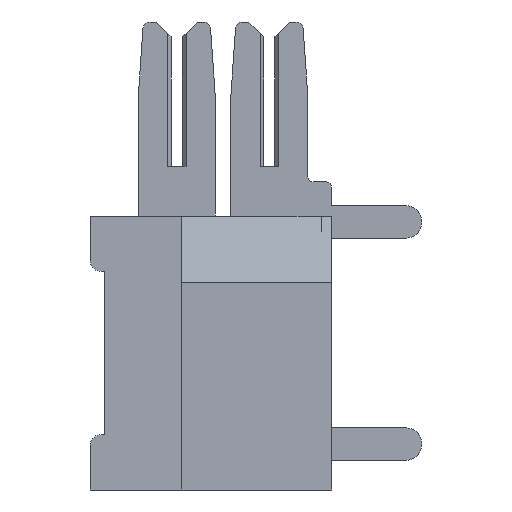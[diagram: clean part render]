
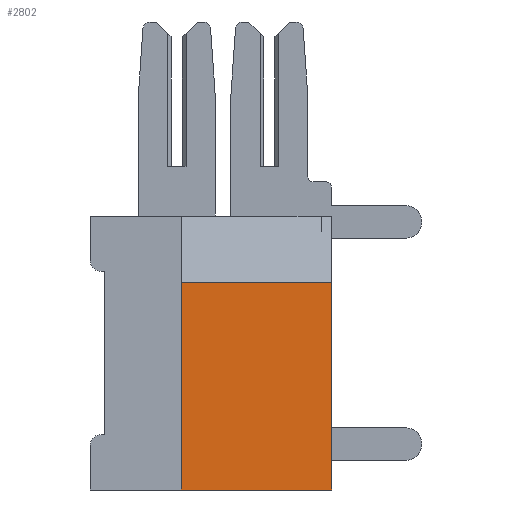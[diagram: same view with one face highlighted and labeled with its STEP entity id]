
A CAD part, left-side view. The second image highlights one B-rep face of the part: STEP entity #2802.
In plain terms, the highlighted planar face has unit normal (-1, 0, 0).
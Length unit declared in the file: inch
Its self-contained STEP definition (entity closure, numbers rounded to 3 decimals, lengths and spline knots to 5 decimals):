
#1 = FACE_OUTER_BOUND ( 'NONE', #800, .T. ) ;
#390 = CARTESIAN_POINT ( 'NONE',  ( 0., 0.326, 0. ) ) ;
#412 = VECTOR ( 'NONE', #3833, 39.37008 ) ;
#800 = EDGE_LOOP ( 'NONE', ( #5650, #11852, #9499, #2534 ) ) ;
#1183 = VERTEX_POINT ( 'NONE', #2715 ) ;
#1211 = EDGE_CURVE ( 'NONE', #10266, #1183, #1977, .T. ) ;
#1630 = DIRECTION ( 'NONE',  ( 0., -1., 0. ) ) ;
#1977 = LINE ( 'NONE', #2856, #8263 ) ;
#2450 = DIRECTION ( 'NONE',  ( 1., 0., 0. ) ) ;
#2514 = LINE ( 'NONE', #2945, #10423 ) ;
#2534 = ORIENTED_EDGE ( 'NONE', *, *, #1211, .T. ) ;
#2715 = CARTESIAN_POINT ( 'NONE',  ( 0., 0., -0.37 ) ) ;
#2802 = ADVANCED_FACE ( 'NONE', ( #1 ), #12447, .F. ) ;
#2856 = CARTESIAN_POINT ( 'NONE',  ( 0., 0.326, -0.37 ) ) ;
#2945 = CARTESIAN_POINT ( 'NONE',  ( 0., 0., -0.09 ) ) ;
#3150 = LINE ( 'NONE', #8929, #412 ) ;
#3765 = AXIS2_PLACEMENT_3D ( 'NONE', #390, #2450, #12671 ) ;
#3833 = DIRECTION ( 'NONE',  ( 0., 0., 1. ) ) ;
#4288 = VERTEX_POINT ( 'NONE', #12915 ) ;
#5051 = DIRECTION ( 'NONE',  ( 0., 1., 0. ) ) ;
#5117 = DIRECTION ( 'NONE',  ( 0., 0., 1. ) ) ;
#5650 = ORIENTED_EDGE ( 'NONE', *, *, #12595, .T. ) ;
#6531 = LINE ( 'NONE', #12086, #11699 ) ;
#7350 = CARTESIAN_POINT ( 'NONE',  ( 0., 0., -0.09 ) ) ;
#8263 = VECTOR ( 'NONE', #1630, 39.37008 ) ;
#8929 = CARTESIAN_POINT ( 'NONE',  ( 0., 0., 0. ) ) ;
#9499 = ORIENTED_EDGE ( 'NONE', *, *, #10853, .F. ) ;
#10266 = VERTEX_POINT ( 'NONE', #12051 ) ;
#10423 = VECTOR ( 'NONE', #5051, 39.37008 ) ;
#10853 = EDGE_CURVE ( 'NONE', #10266, #4288, #6531, .T. ) ;
#11482 = EDGE_CURVE ( 'NONE', #12166, #4288, #2514, .T. ) ;
#11699 = VECTOR ( 'NONE', #5117, 39.37008 ) ;
#11852 = ORIENTED_EDGE ( 'NONE', *, *, #11482, .T. ) ;
#12051 = CARTESIAN_POINT ( 'NONE',  ( 0., 0.203, -0.37 ) ) ;
#12086 = CARTESIAN_POINT ( 'NONE',  ( 0., 0.203, -0.37 ) ) ;
#12166 = VERTEX_POINT ( 'NONE', #7350 ) ;
#12447 = PLANE ( 'NONE',  #3765 ) ;
#12595 = EDGE_CURVE ( 'NONE', #1183, #12166, #3150, .T. ) ;
#12671 = DIRECTION ( 'NONE',  ( 0., 0., -1. ) ) ;
#12915 = CARTESIAN_POINT ( 'NONE',  ( 0., 0.203, -0.09 ) ) ;
